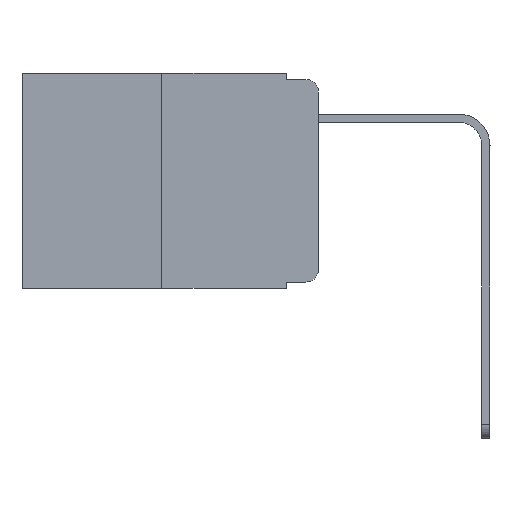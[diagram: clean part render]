
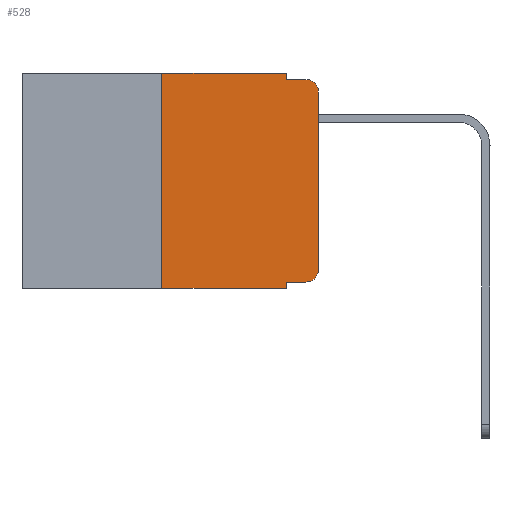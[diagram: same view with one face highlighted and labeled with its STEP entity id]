
A CAD part, left-side view. The second image highlights one B-rep face of the part: STEP entity #528.
In plain terms, the highlighted planar face has unit normal (-1, 0, 0).
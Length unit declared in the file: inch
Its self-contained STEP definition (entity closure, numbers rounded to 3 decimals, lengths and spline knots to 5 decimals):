
#38 = VECTOR ( 'NONE', #9105, 39.37008 ) ;
#252 = LINE ( 'NONE', #10363, #20594 ) ;
#528 = ADVANCED_FACE ( 'NONE', ( #3776 ), #3801, .F. ) ;
#1452 = CARTESIAN_POINT ( 'NONE',  ( 0., 0., -0.313 ) ) ;
#1703 = DIRECTION ( 'NONE',  ( 0., -1., 0. ) ) ;
#2058 = EDGE_CURVE ( 'NONE', #16296, #7610, #12307, .T. ) ;
#2079 = LINE ( 'NONE', #12458, #12876 ) ;
#3171 = CARTESIAN_POINT ( 'NONE',  ( 0., 0.02, -0.333 ) ) ;
#3218 = VERTEX_POINT ( 'NONE', #14212 ) ;
#3239 = LINE ( 'NONE', #3698, #10358 ) ;
#3360 = VECTOR ( 'NONE', #22340, 39.37008 ) ;
#3698 = CARTESIAN_POINT ( 'NONE',  ( 0., 0.25, 0. ) ) ;
#3776 = FACE_OUTER_BOUND ( 'NONE', #20588, .T. ) ;
#3801 = PLANE ( 'NONE',  #11349 ) ;
#4339 = ORIENTED_EDGE ( 'NONE', *, *, #13818, .F. ) ;
#4674 = EDGE_CURVE ( 'NONE', #21530, #21209, #12847, .T. ) ;
#5123 = VERTEX_POINT ( 'NONE', #3171 ) ;
#5183 = ORIENTED_EDGE ( 'NONE', *, *, #16499, .T. ) ;
#5306 = CARTESIAN_POINT ( 'NONE',  ( 0., 0.473, -0.343 ) ) ;
#5955 = CARTESIAN_POINT ( 'NONE',  ( 0., 0.473, 0. ) ) ;
#6118 = LINE ( 'NONE', #13481, #16291 ) ;
#6450 = DIRECTION ( 'NONE',  ( 0., -1., 0. ) ) ;
#6910 = CARTESIAN_POINT ( 'NONE',  ( 0., 0.051, -0.333 ) ) ;
#7610 = VERTEX_POINT ( 'NONE', #23533 ) ;
#7701 = CARTESIAN_POINT ( 'NONE',  ( 0., 0.02, -0.313 ) ) ;
#7942 = DIRECTION ( 'NONE',  ( 0., 0., -1. ) ) ;
#9091 = ORIENTED_EDGE ( 'NONE', *, *, #9387, .F. ) ;
#9105 = DIRECTION ( 'NONE',  ( 0., -1., 0. ) ) ;
#9387 = EDGE_CURVE ( 'NONE', #13483, #24784, #3239, .T. ) ;
#10358 = VECTOR ( 'NONE', #13541, 39.37008 ) ;
#10363 = CARTESIAN_POINT ( 'NONE',  ( 0., 0.473, 0. ) ) ;
#10444 = LINE ( 'NONE', #12210, #15038 ) ;
#11349 = AXIS2_PLACEMENT_3D ( 'NONE', #5955, #21658, #7942 ) ;
#11642 = DIRECTION ( 'NONE',  ( 0., 0., -1. ) ) ;
#11670 = ORIENTED_EDGE ( 'NONE', *, *, #2058, .F. ) ;
#11870 = ORIENTED_EDGE ( 'NONE', *, *, #22890, .F. ) ;
#12210 = CARTESIAN_POINT ( 'NONE',  ( 0., 0.051, 0. ) ) ;
#12307 = LINE ( 'NONE', #20336, #3360 ) ;
#12458 = CARTESIAN_POINT ( 'NONE',  ( 0., 0.051, -0.333 ) ) ;
#12685 = ORIENTED_EDGE ( 'NONE', *, *, #4674, .T. ) ;
#12847 = CIRCLE ( 'NONE', #17654, 0.02 ) ;
#12876 = VECTOR ( 'NONE', #24027, 39.37008 ) ;
#13326 = AXIS2_PLACEMENT_3D ( 'NONE', #7701, #19579, #17445 ) ;
#13333 = VECTOR ( 'NONE', #15498, 39.37008 ) ;
#13481 = CARTESIAN_POINT ( 'NONE',  ( 0., 0.051, -0.01 ) ) ;
#13483 = VERTEX_POINT ( 'NONE', #14900 ) ;
#13503 = ORIENTED_EDGE ( 'NONE', *, *, #17618, .F. ) ;
#13541 = DIRECTION ( 'NONE',  ( 0., 0., 1. ) ) ;
#13818 = EDGE_CURVE ( 'NONE', #25483, #3218, #10444, .T. ) ;
#13952 = EDGE_CURVE ( 'NONE', #25483, #5123, #2079, .T. ) ;
#14212 = CARTESIAN_POINT ( 'NONE',  ( 0., 0.051, -0.343 ) ) ;
#14214 = EDGE_CURVE ( 'NONE', #5123, #21177, #20877, .T. ) ;
#14822 = ORIENTED_EDGE ( 'NONE', *, *, #20102, .T. ) ;
#14900 = CARTESIAN_POINT ( 'NONE',  ( 0., 0.25, -0.343 ) ) ;
#15038 = VECTOR ( 'NONE', #16270, 39.37008 ) ;
#15498 = DIRECTION ( 'NONE',  ( 0., 0., 1. ) ) ;
#15924 = CARTESIAN_POINT ( 'NONE',  ( 0., 0.051, 0. ) ) ;
#16270 = DIRECTION ( 'NONE',  ( 0., 0., -1. ) ) ;
#16291 = VECTOR ( 'NONE', #1703, 39.37008 ) ;
#16296 = VERTEX_POINT ( 'NONE', #15924 ) ;
#16344 = CARTESIAN_POINT ( 'NONE',  ( 0., 0., -0.03 ) ) ;
#16499 = EDGE_CURVE ( 'NONE', #13483, #3218, #19739, .T. ) ;
#16779 = LINE ( 'NONE', #21274, #13333 ) ;
#17445 = DIRECTION ( 'NONE',  ( 0., 0., -1. ) ) ;
#17618 = EDGE_CURVE ( 'NONE', #24784, #16296, #252, .T. ) ;
#17654 = AXIS2_PLACEMENT_3D ( 'NONE', #25518, #19712, #11642 ) ;
#18122 = ORIENTED_EDGE ( 'NONE', *, *, #14214, .T. ) ;
#18293 = CARTESIAN_POINT ( 'NONE',  ( 0., 0.25, 0. ) ) ;
#19574 = ORIENTED_EDGE ( 'NONE', *, *, #13952, .T. ) ;
#19579 = DIRECTION ( 'NONE',  ( -1., 0., 0. ) ) ;
#19712 = DIRECTION ( 'NONE',  ( -1., 0., 0. ) ) ;
#19739 = LINE ( 'NONE', #5306, #38 ) ;
#20102 = EDGE_CURVE ( 'NONE', #21177, #21530, #16779, .T. ) ;
#20336 = CARTESIAN_POINT ( 'NONE',  ( 0., 0.051, 0. ) ) ;
#20588 = EDGE_LOOP ( 'NONE', ( #14822, #12685, #11870, #11670, #13503, #9091, #5183, #4339, #19574, #18122 ) ) ;
#20594 = VECTOR ( 'NONE', #6450, 39.37008 ) ;
#20877 = CIRCLE ( 'NONE', #13326, 0.02 ) ;
#21177 = VERTEX_POINT ( 'NONE', #1452 ) ;
#21209 = VERTEX_POINT ( 'NONE', #25153 ) ;
#21274 = CARTESIAN_POINT ( 'NONE',  ( 0., 0., 0. ) ) ;
#21530 = VERTEX_POINT ( 'NONE', #16344 ) ;
#21658 = DIRECTION ( 'NONE',  ( 1., 0., 0. ) ) ;
#22340 = DIRECTION ( 'NONE',  ( 0., 0., -1. ) ) ;
#22890 = EDGE_CURVE ( 'NONE', #7610, #21209, #6118, .T. ) ;
#23533 = CARTESIAN_POINT ( 'NONE',  ( 0., 0.051, -0.01 ) ) ;
#24027 = DIRECTION ( 'NONE',  ( 0., -1., 0. ) ) ;
#24784 = VERTEX_POINT ( 'NONE', #18293 ) ;
#25153 = CARTESIAN_POINT ( 'NONE',  ( 0., 0.02, -0.01 ) ) ;
#25483 = VERTEX_POINT ( 'NONE', #6910 ) ;
#25518 = CARTESIAN_POINT ( 'NONE',  ( 0., 0.02, -0.03 ) ) ;
